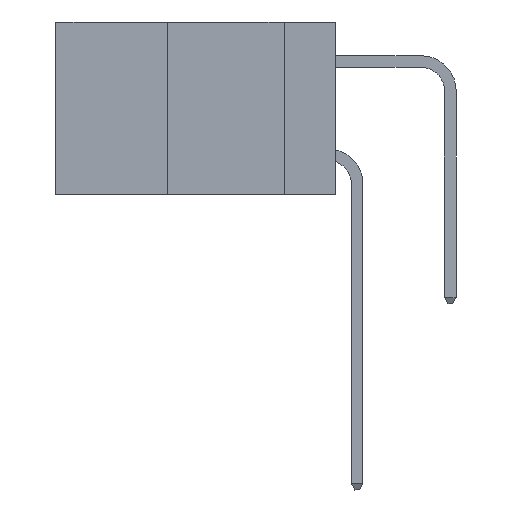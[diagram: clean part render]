
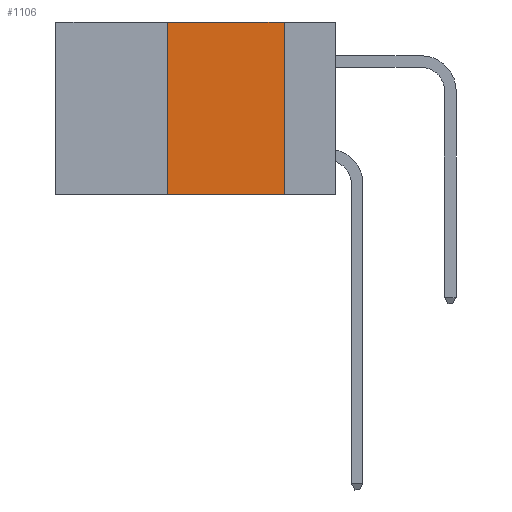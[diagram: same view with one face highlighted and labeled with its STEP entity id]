
A CAD part, left-side view. The second image highlights one B-rep face of the part: STEP entity #1106.
In plain terms, the highlighted planar face has unit normal (-1, 0, 0).
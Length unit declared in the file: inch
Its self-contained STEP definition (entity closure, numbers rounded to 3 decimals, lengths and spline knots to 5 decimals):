
#410 = DIRECTION ( 'NONE',  ( 0., 0., -1. ) ) ;
#419 = CARTESIAN_POINT ( 'NONE',  ( 0., 0.6, 0. ) ) ;
#706 = EDGE_LOOP ( 'NONE', ( #19095, #14006, #19289, #24887 ) ) ;
#1106 = ADVANCED_FACE ( 'NONE', ( #17593 ), #5650, .F. ) ;
#2647 = CARTESIAN_POINT ( 'NONE',  ( 0., 0.11, 0. ) ) ;
#3161 = EDGE_CURVE ( 'NONE', #20467, #6575, #8328, .T. ) ;
#3423 = EDGE_CURVE ( 'NONE', #6575, #4863, #7257, .T. ) ;
#4633 = CARTESIAN_POINT ( 'NONE',  ( 0., 0.11, -0.37 ) ) ;
#4863 = VERTEX_POINT ( 'NONE', #2647 ) ;
#5518 = VECTOR ( 'NONE', #410, 39.37008 ) ;
#5555 = CARTESIAN_POINT ( 'NONE',  ( 0., 0.6, 0. ) ) ;
#5650 = PLANE ( 'NONE',  #17029 ) ;
#6002 = VERTEX_POINT ( 'NONE', #4633 ) ;
#6413 = CARTESIAN_POINT ( 'NONE',  ( 0., 0.36, 0. ) ) ;
#6575 = VERTEX_POINT ( 'NONE', #6413 ) ;
#7257 = LINE ( 'NONE', #419, #25623 ) ;
#7261 = VECTOR ( 'NONE', #23796, 39.37008 ) ;
#8328 = LINE ( 'NONE', #26498, #27376 ) ;
#8659 = LINE ( 'NONE', #21592, #7261 ) ;
#9628 = DIRECTION ( 'NONE',  ( 0., -1., 0. ) ) ;
#12766 = LINE ( 'NONE', #24904, #5518 ) ;
#14006 = ORIENTED_EDGE ( 'NONE', *, *, #3423, .F. ) ;
#15472 = CARTESIAN_POINT ( 'NONE',  ( 0., 0.36, -0.37 ) ) ;
#16953 = DIRECTION ( 'NONE',  ( 1., 0., 0. ) ) ;
#17029 = AXIS2_PLACEMENT_3D ( 'NONE', #5555, #16953, #23445 ) ;
#17593 = FACE_OUTER_BOUND ( 'NONE', #706, .T. ) ;
#17902 = DIRECTION ( 'NONE',  ( 0., 0., 1. ) ) ;
#19095 = ORIENTED_EDGE ( 'NONE', *, *, #21986, .F. ) ;
#19289 = ORIENTED_EDGE ( 'NONE', *, *, #3161, .F. ) ;
#20467 = VERTEX_POINT ( 'NONE', #15472 ) ;
#21592 = CARTESIAN_POINT ( 'NONE',  ( 0., 0.6, -0.37 ) ) ;
#21986 = EDGE_CURVE ( 'NONE', #4863, #6002, #12766, .T. ) ;
#23445 = DIRECTION ( 'NONE',  ( 0., 0., -1. ) ) ;
#23796 = DIRECTION ( 'NONE',  ( 0., -1., 0. ) ) ;
#24887 = ORIENTED_EDGE ( 'NONE', *, *, #28425, .T. ) ;
#24904 = CARTESIAN_POINT ( 'NONE',  ( 0., 0.11, 0. ) ) ;
#25623 = VECTOR ( 'NONE', #9628, 39.37008 ) ;
#26498 = CARTESIAN_POINT ( 'NONE',  ( 0., 0.36, 0. ) ) ;
#27376 = VECTOR ( 'NONE', #17902, 39.37008 ) ;
#28425 = EDGE_CURVE ( 'NONE', #20467, #6002, #8659, .T. ) ;
